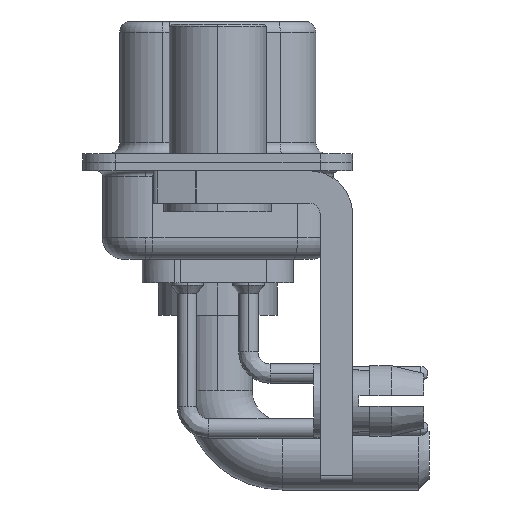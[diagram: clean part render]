
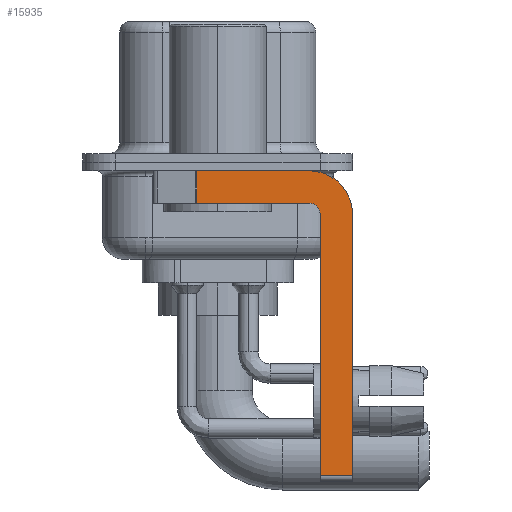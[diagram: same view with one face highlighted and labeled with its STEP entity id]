
A CAD part, left-side view. The second image highlights one B-rep face of the part: STEP entity #15935.
In plain terms, the highlighted planar face has unit normal (-1, 0, 0).
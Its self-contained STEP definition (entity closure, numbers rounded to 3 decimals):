
#8 = ORIENTED_EDGE ( 'NONE', *, *, #16406, .F. ) ;
#510 = LINE ( 'NONE', #14503, #14239 ) ;
#1122 = LINE ( 'NONE', #8317, #4612 ) ;
#1272 = CARTESIAN_POINT ( 'NONE',  ( -2.9, -4.25, -2.4 ) ) ;
#1568 = AXIS2_PLACEMENT_3D ( 'NONE', #1272, #6842, #4780 ) ;
#2215 = VECTOR ( 'NONE', #13618, 1000. ) ;
#2988 = CARTESIAN_POINT ( 'NONE',  ( -2.9, 3., -0.4 ) ) ;
#3017 = LINE ( 'NONE', #15378, #20038 ) ;
#3338 = AXIS2_PLACEMENT_3D ( 'NONE', #13764, #12481, #19539 ) ;
#3783 = ORIENTED_EDGE ( 'NONE', *, *, #11839, .F. ) ;
#4018 = ORIENTED_EDGE ( 'NONE', *, *, #20075, .F. ) ;
#4612 = VECTOR ( 'NONE', #8091, 1000. ) ;
#4780 = DIRECTION ( 'NONE',  ( 0., 0., -1. ) ) ;
#4966 = LINE ( 'NONE', #18718, #2215 ) ;
#5159 = VERTEX_POINT ( 'NONE', #11008 ) ;
#5230 = DIRECTION ( 'NONE',  ( 0., 0., -1. ) ) ;
#6256 = EDGE_CURVE ( 'NONE', #7046, #12363, #4966, .T. ) ;
#6315 = CARTESIAN_POINT ( 'NONE',  ( -2.9, -4.25, -0.4 ) ) ;
#6331 = VERTEX_POINT ( 'NONE', #8542 ) ;
#6493 = FACE_OUTER_BOUND ( 'NONE', #15967, .T. ) ;
#6842 = DIRECTION ( 'NONE',  ( 1., 0., 0. ) ) ;
#7046 = VERTEX_POINT ( 'NONE', #20201 ) ;
#7320 = VERTEX_POINT ( 'NONE', #20405 ) ;
#8091 = DIRECTION ( 'NONE',  ( 0., -1., 0. ) ) ;
#8235 = EDGE_CURVE ( 'NONE', #6331, #19239, #510, .T. ) ;
#8317 = CARTESIAN_POINT ( 'NONE',  ( -2.9, -4.25, -14.55 ) ) ;
#8542 = CARTESIAN_POINT ( 'NONE',  ( -2.9, -4.25, -1.9 ) ) ;
#9178 = VECTOR ( 'NONE', #17097, 1000. ) ;
#9468 = CARTESIAN_POINT ( 'NONE',  ( -2.9, -4.75, -2.4 ) ) ;
#9703 = EDGE_CURVE ( 'NONE', #7046, #5159, #1122, .T. ) ;
#9924 = CARTESIAN_POINT ( 'NONE',  ( -2.9, -4.25, -2.4 ) ) ;
#10071 = LINE ( 'NONE', #17128, #11501 ) ;
#10145 = ORIENTED_EDGE ( 'NONE', *, *, #8235, .F. ) ;
#11008 = CARTESIAN_POINT ( 'NONE',  ( -2.9, -6.25, -14.55 ) ) ;
#11501 = VECTOR ( 'NONE', #5230, 1000. ) ;
#11839 = EDGE_CURVE ( 'NONE', #14025, #7320, #21403, .T. ) ;
#11926 = PLANE ( 'NONE',  #1568 ) ;
#12363 = VERTEX_POINT ( 'NONE', #9468 ) ;
#12481 = DIRECTION ( 'NONE',  ( 1., 0., 0. ) ) ;
#13513 = DIRECTION ( 'NONE',  ( 0., 0., 1. ) ) ;
#13573 = CARTESIAN_POINT ( 'NONE',  ( -2.9, 0.978, -1.9 ) ) ;
#13618 = DIRECTION ( 'NONE',  ( 0., 0., 1. ) ) ;
#13679 = EDGE_CURVE ( 'NONE', #7320, #5159, #10071, .T. ) ;
#13764 = CARTESIAN_POINT ( 'NONE',  ( -2.9, -4.25, -2.4 ) ) ;
#14025 = VERTEX_POINT ( 'NONE', #6315 ) ;
#14239 = VECTOR ( 'NONE', #15898, 1000. ) ;
#14503 = CARTESIAN_POINT ( 'NONE',  ( -2.9, -4.25, -1.9 ) ) ;
#14532 = ORIENTED_EDGE ( 'NONE', *, *, #13679, .F. ) ;
#15378 = CARTESIAN_POINT ( 'NONE',  ( -2.9, 0.978, -1.9 ) ) ;
#15894 = EDGE_CURVE ( 'NONE', #22063, #19239, #3017, .T. ) ;
#15898 = DIRECTION ( 'NONE',  ( 0., 1., 0. ) ) ;
#15935 = ADVANCED_FACE ( 'NONE', ( #6493 ), #11926, .F. ) ;
#15967 = EDGE_LOOP ( 'NONE', ( #8, #16573, #10145, #4018, #18223, #16619, #14532, #3783 ) ) ;
#16406 = EDGE_CURVE ( 'NONE', #22063, #14025, #18837, .T. ) ;
#16573 = ORIENTED_EDGE ( 'NONE', *, *, #15894, .T. ) ;
#16619 = ORIENTED_EDGE ( 'NONE', *, *, #9703, .T. ) ;
#17097 = DIRECTION ( 'NONE',  ( 0., -1., 0. ) ) ;
#17128 = CARTESIAN_POINT ( 'NONE',  ( -2.9, -6.25, -2.4 ) ) ;
#17494 = AXIS2_PLACEMENT_3D ( 'NONE', #9924, #18614, #13513 ) ;
#18223 = ORIENTED_EDGE ( 'NONE', *, *, #6256, .F. ) ;
#18555 = CARTESIAN_POINT ( 'NONE',  ( -2.9, 0.978, -0.4 ) ) ;
#18614 = DIRECTION ( 'NONE',  ( -1., 0., 0. ) ) ;
#18718 = CARTESIAN_POINT ( 'NONE',  ( -2.9, -4.75, -14.8 ) ) ;
#18837 = LINE ( 'NONE', #2988, #9178 ) ;
#19239 = VERTEX_POINT ( 'NONE', #13573 ) ;
#19539 = DIRECTION ( 'NONE',  ( 0., 0., -1. ) ) ;
#20038 = VECTOR ( 'NONE', #20830, 1000. ) ;
#20075 = EDGE_CURVE ( 'NONE', #12363, #6331, #20819, .T. ) ;
#20201 = CARTESIAN_POINT ( 'NONE',  ( -2.9, -4.75, -14.55 ) ) ;
#20405 = CARTESIAN_POINT ( 'NONE',  ( -2.9, -6.25, -2.4 ) ) ;
#20819 = CIRCLE ( 'NONE', #17494, 0.5 ) ;
#20830 = DIRECTION ( 'NONE',  ( 0., 0., -1. ) ) ;
#21403 = CIRCLE ( 'NONE', #3338, 2. ) ;
#22063 = VERTEX_POINT ( 'NONE', #18555 ) ;
